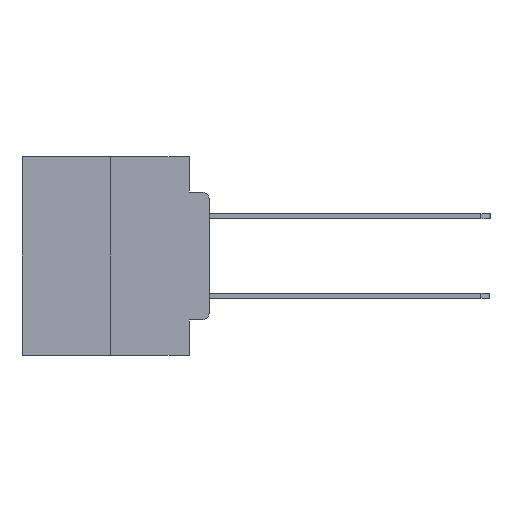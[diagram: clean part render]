
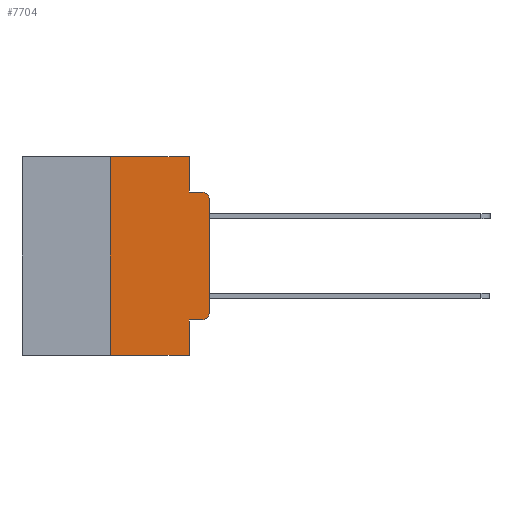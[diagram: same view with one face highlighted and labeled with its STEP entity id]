
A CAD part, left-side view. The second image highlights one B-rep face of the part: STEP entity #7704.
In plain terms, the highlighted planar face has unit normal (-1, 0, 0).
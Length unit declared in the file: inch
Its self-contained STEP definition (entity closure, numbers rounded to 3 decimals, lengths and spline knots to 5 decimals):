
#349 = VECTOR ( 'NONE', #25617, 39.37008 ) ;
#715 = EDGE_CURVE ( 'NONE', #16607, #22796, #11066, .T. ) ;
#1390 = VERTEX_POINT ( 'NONE', #13768 ) ;
#1590 = CARTESIAN_POINT ( 'NONE',  ( 0., 0.051, -0.4115 ) ) ;
#2300 = ORIENTED_EDGE ( 'NONE', *, *, #17085, .T. ) ;
#2723 = CARTESIAN_POINT ( 'NONE',  ( 0., 0.02, -0.4115 ) ) ;
#2772 = DIRECTION ( 'NONE',  ( 0., -1., 0. ) ) ;
#2873 = CARTESIAN_POINT ( 'NONE',  ( 0., 0.473, 0. ) ) ;
#3044 = DIRECTION ( 'NONE',  ( 0., -1., 0. ) ) ;
#3396 = CARTESIAN_POINT ( 'NONE',  ( 0., 0.051, 0. ) ) ;
#5163 = ORIENTED_EDGE ( 'NONE', *, *, #14333, .T. ) ;
#5256 = DIRECTION ( 'NONE',  ( -1., 0., 0. ) ) ;
#5718 = VERTEX_POINT ( 'NONE', #24603 ) ;
#5812 = CARTESIAN_POINT ( 'NONE',  ( 0., 0.473, 0. ) ) ;
#6039 = VECTOR ( 'NONE', #10850, 39.37008 ) ;
#6339 = CARTESIAN_POINT ( 'NONE',  ( 0., 0.25, 0. ) ) ;
#6576 = EDGE_CURVE ( 'NONE', #20123, #16607, #18327, .T. ) ;
#6801 = VECTOR ( 'NONE', #16890, 39.37008 ) ;
#6839 = CARTESIAN_POINT ( 'NONE',  ( 0., 0.02, -0.1085 ) ) ;
#6909 = DIRECTION ( 'NONE',  ( 0., -1., 0. ) ) ;
#7019 = LINE ( 'NONE', #11549, #12345 ) ;
#7681 = CARTESIAN_POINT ( 'NONE',  ( 0., 0.02, -0.0885 ) ) ;
#7704 = ADVANCED_FACE ( 'NONE', ( #27226 ), #19222, .F. ) ;
#8261 = ORIENTED_EDGE ( 'NONE', *, *, #15603, .T. ) ;
#8517 = CARTESIAN_POINT ( 'NONE',  ( 0., 0., 0. ) ) ;
#9141 = DIRECTION ( 'NONE',  ( 0., 0., -1. ) ) ;
#9209 = CARTESIAN_POINT ( 'NONE',  ( 0., 0.473, -0.5 ) ) ;
#9413 = VERTEX_POINT ( 'NONE', #2723 ) ;
#9438 = VECTOR ( 'NONE', #24066, 39.37008 ) ;
#9615 = EDGE_CURVE ( 'NONE', #22796, #1390, #18715, .T. ) ;
#9824 = CARTESIAN_POINT ( 'NONE',  ( 0., 0.051, -0.0885 ) ) ;
#10379 = DIRECTION ( 'NONE',  ( 0., 0., -1. ) ) ;
#10850 = DIRECTION ( 'NONE',  ( 0., -1., 0. ) ) ;
#11066 = LINE ( 'NONE', #2873, #22164 ) ;
#11142 = EDGE_CURVE ( 'NONE', #1390, #22992, #26200, .T. ) ;
#11549 = CARTESIAN_POINT ( 'NONE',  ( 0., 0.051, 0. ) ) ;
#11944 = ORIENTED_EDGE ( 'NONE', *, *, #25045, .T. ) ;
#12345 = VECTOR ( 'NONE', #15998, 39.37008 ) ;
#12384 = CARTESIAN_POINT ( 'NONE',  ( 0., 0.25, 0. ) ) ;
#12773 = LINE ( 'NONE', #1590, #6039 ) ;
#13768 = CARTESIAN_POINT ( 'NONE',  ( 0., 0.051, -0.0885 ) ) ;
#14333 = EDGE_CURVE ( 'NONE', #20123, #20596, #18473, .T. ) ;
#14681 = LINE ( 'NONE', #8517, #9438 ) ;
#15603 = EDGE_CURVE ( 'NONE', #21528, #22992, #24807, .T. ) ;
#15998 = DIRECTION ( 'NONE',  ( 0., 0., -1. ) ) ;
#16607 = VERTEX_POINT ( 'NONE', #6339 ) ;
#16890 = DIRECTION ( 'NONE',  ( 0., 0., -1. ) ) ;
#17085 = EDGE_CURVE ( 'NONE', #5718, #21528, #14681, .T. ) ;
#18327 = LINE ( 'NONE', #12384, #349 ) ;
#18473 = LINE ( 'NONE', #9209, #23638 ) ;
#18702 = CARTESIAN_POINT ( 'NONE',  ( 0., 0.02, -0.3915 ) ) ;
#18715 = LINE ( 'NONE', #3396, #6801 ) ;
#19222 = PLANE ( 'NONE',  #27183 ) ;
#20123 = VERTEX_POINT ( 'NONE', #22148 ) ;
#20342 = VECTOR ( 'NONE', #3044, 39.37008 ) ;
#20374 = CARTESIAN_POINT ( 'NONE',  ( 0., 0.051, 0. ) ) ;
#20561 = AXIS2_PLACEMENT_3D ( 'NONE', #6839, #22451, #9141 ) ;
#20596 = VERTEX_POINT ( 'NONE', #26264 ) ;
#20724 = CARTESIAN_POINT ( 'NONE',  ( 0., 0., -0.1085 ) ) ;
#20869 = ORIENTED_EDGE ( 'NONE', *, *, #715, .F. ) ;
#20927 = DIRECTION ( 'NONE',  ( 0., 0., -1. ) ) ;
#21528 = VERTEX_POINT ( 'NONE', #20724 ) ;
#21594 = EDGE_LOOP ( 'NONE', ( #2300, #8261, #22197, #24274, #20869, #23625, #5163, #21971, #11944, #25773 ) ) ;
#21971 = ORIENTED_EDGE ( 'NONE', *, *, #27978, .F. ) ;
#22148 = CARTESIAN_POINT ( 'NONE',  ( 0., 0.25, -0.5 ) ) ;
#22164 = VECTOR ( 'NONE', #2772, 39.37008 ) ;
#22197 = ORIENTED_EDGE ( 'NONE', *, *, #11142, .F. ) ;
#22451 = DIRECTION ( 'NONE',  ( -1., 0., 0. ) ) ;
#22796 = VERTEX_POINT ( 'NONE', #20374 ) ;
#22866 = CARTESIAN_POINT ( 'NONE',  ( 0., 0.051, -0.4115 ) ) ;
#22992 = VERTEX_POINT ( 'NONE', #7681 ) ;
#23554 = EDGE_CURVE ( 'NONE', #9413, #5718, #28718, .T. ) ;
#23625 = ORIENTED_EDGE ( 'NONE', *, *, #6576, .F. ) ;
#23638 = VECTOR ( 'NONE', #6909, 39.37008 ) ;
#23662 = DIRECTION ( 'NONE',  ( 1., 0., 0. ) ) ;
#24066 = DIRECTION ( 'NONE',  ( 0., 0., 1. ) ) ;
#24274 = ORIENTED_EDGE ( 'NONE', *, *, #9615, .F. ) ;
#24603 = CARTESIAN_POINT ( 'NONE',  ( 0., 0., -0.3915 ) ) ;
#24807 = CIRCLE ( 'NONE', #20561, 0.02 ) ;
#25045 = EDGE_CURVE ( 'NONE', #25303, #9413, #12773, .T. ) ;
#25303 = VERTEX_POINT ( 'NONE', #22866 ) ;
#25617 = DIRECTION ( 'NONE',  ( 0., 0., 1. ) ) ;
#25773 = ORIENTED_EDGE ( 'NONE', *, *, #23554, .T. ) ;
#26200 = LINE ( 'NONE', #9824, #20342 ) ;
#26264 = CARTESIAN_POINT ( 'NONE',  ( 0., 0.051, -0.5 ) ) ;
#27183 = AXIS2_PLACEMENT_3D ( 'NONE', #5812, #23662, #10379 ) ;
#27226 = FACE_OUTER_BOUND ( 'NONE', #21594, .T. ) ;
#27881 = AXIS2_PLACEMENT_3D ( 'NONE', #18702, #5256, #20927 ) ;
#27978 = EDGE_CURVE ( 'NONE', #25303, #20596, #7019, .T. ) ;
#28718 = CIRCLE ( 'NONE', #27881, 0.02 ) ;
